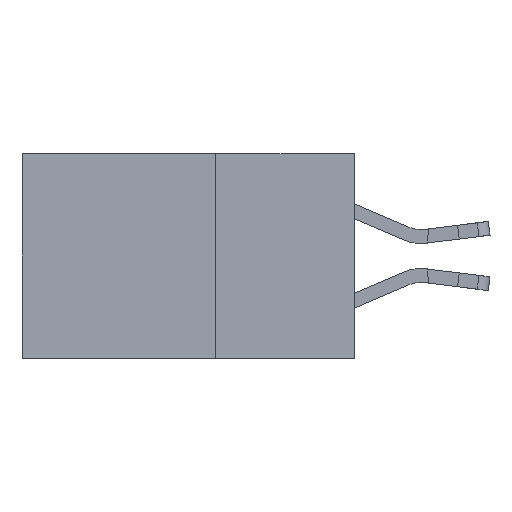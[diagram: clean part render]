
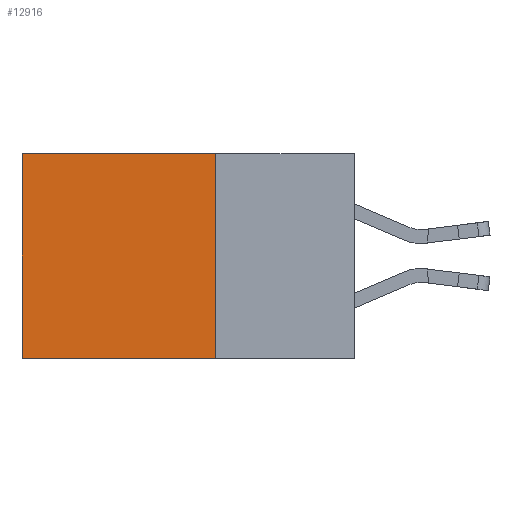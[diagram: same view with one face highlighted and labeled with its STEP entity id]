
A CAD part, left-side view. The second image highlights one B-rep face of the part: STEP entity #12916.
In plain terms, the highlighted planar face has unit normal (-1, 0, 0).
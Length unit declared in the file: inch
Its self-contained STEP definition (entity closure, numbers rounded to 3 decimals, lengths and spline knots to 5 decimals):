
#89 = ORIENTED_EDGE ( 'NONE', *, *, #3023, .T. ) ;
#923 = CARTESIAN_POINT ( 'NONE',  ( 0.298, 0.6, -0.37 ) ) ;
#1072 = VECTOR ( 'NONE', #1735, 39.37008 ) ;
#1628 = CARTESIAN_POINT ( 'NONE',  ( 0.298, 0.6, 0. ) ) ;
#1735 = DIRECTION ( 'NONE',  ( 0., 0., -1. ) ) ;
#1813 = LINE ( 'NONE', #1628, #1072 ) ;
#3023 = EDGE_CURVE ( 'NONE', #8311, #10630, #10763, .T. ) ;
#3468 = ORIENTED_EDGE ( 'NONE', *, *, #13093, .F. ) ;
#3633 = DIRECTION ( 'NONE',  ( 0., 1., 0. ) ) ;
#5171 = CARTESIAN_POINT ( 'NONE',  ( 0.298, 0.25, -0.37 ) ) ;
#5176 = LINE ( 'NONE', #11490, #13823 ) ;
#5309 = LINE ( 'NONE', #10505, #8375 ) ;
#5558 = DIRECTION ( 'NONE',  ( 1., 0., 0. ) ) ;
#6369 = VERTEX_POINT ( 'NONE', #5171 ) ;
#6432 = EDGE_CURVE ( 'NONE', #10630, #13564, #1813, .T. ) ;
#6593 = CARTESIAN_POINT ( 'NONE',  ( 0.298, 0.6, 0. ) ) ;
#7381 = ORIENTED_EDGE ( 'NONE', *, *, #6432, .T. ) ;
#7756 = ORIENTED_EDGE ( 'NONE', *, *, #14596, .F. ) ;
#8113 = DIRECTION ( 'NONE',  ( 0., 0., -1. ) ) ;
#8286 = DIRECTION ( 'NONE',  ( 0., 1., 0. ) ) ;
#8311 = VERTEX_POINT ( 'NONE', #12316 ) ;
#8375 = VECTOR ( 'NONE', #3633, 39.37008 ) ;
#8925 = FACE_OUTER_BOUND ( 'NONE', #12415, .T. ) ;
#10505 = CARTESIAN_POINT ( 'NONE',  ( 0.298, 0.25, -0.37 ) ) ;
#10630 = VERTEX_POINT ( 'NONE', #6593 ) ;
#10763 = LINE ( 'NONE', #12207, #11124 ) ;
#11124 = VECTOR ( 'NONE', #8286, 39.37008 ) ;
#11490 = CARTESIAN_POINT ( 'NONE',  ( 0.298, 0.25, 0. ) ) ;
#12207 = CARTESIAN_POINT ( 'NONE',  ( 0.298, 0.25, 0. ) ) ;
#12316 = CARTESIAN_POINT ( 'NONE',  ( 0.298, 0.25, 0. ) ) ;
#12318 = CARTESIAN_POINT ( 'NONE',  ( 0.298, 0.25, 0. ) ) ;
#12371 = PLANE ( 'NONE',  #12671 ) ;
#12415 = EDGE_LOOP ( 'NONE', ( #7381, #3468, #7756, #89 ) ) ;
#12671 = AXIS2_PLACEMENT_3D ( 'NONE', #12318, #5558, #13456 ) ;
#12916 = ADVANCED_FACE ( 'NONE', ( #8925 ), #12371, .F. ) ;
#13093 = EDGE_CURVE ( 'NONE', #6369, #13564, #5309, .T. ) ;
#13456 = DIRECTION ( 'NONE',  ( 0., 0., -1. ) ) ;
#13564 = VERTEX_POINT ( 'NONE', #923 ) ;
#13823 = VECTOR ( 'NONE', #8113, 39.37008 ) ;
#14596 = EDGE_CURVE ( 'NONE', #8311, #6369, #5176, .T. ) ;
